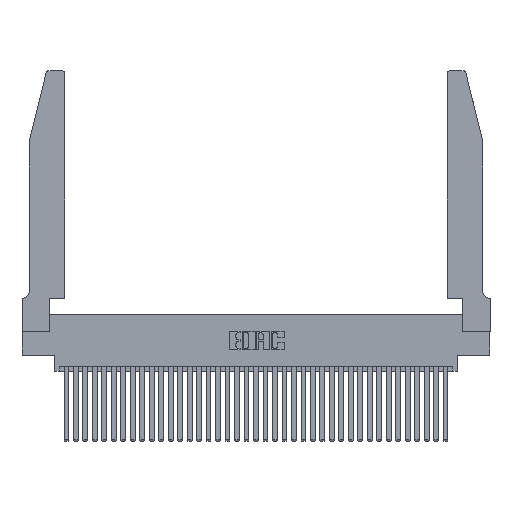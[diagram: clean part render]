
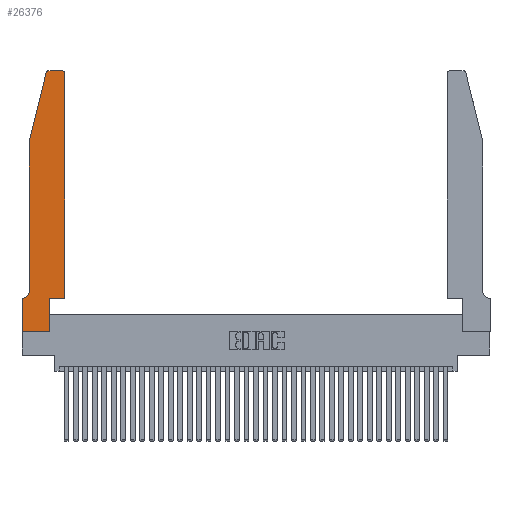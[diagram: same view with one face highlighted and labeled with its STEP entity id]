
A CAD part, top view. The second image highlights one B-rep face of the part: STEP entity #26376.
In plain terms, the highlighted planar face has unit normal (0, 0, 1).
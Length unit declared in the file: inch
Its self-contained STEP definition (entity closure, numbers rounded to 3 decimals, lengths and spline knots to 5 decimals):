
#1013 = VERTEX_POINT ( 'NONE', #22305 ) ;
#1268 = ORIENTED_EDGE ( 'NONE', *, *, #36997, .T. ) ;
#1729 = VERTEX_POINT ( 'NONE', #36439 ) ;
#1864 = DIRECTION ( 'NONE',  ( 0., 0., 1. ) ) ;
#2019 = EDGE_CURVE ( 'NONE', #1013, #4661, #13661, .T. ) ;
#2986 = VERTEX_POINT ( 'NONE', #23632 ) ;
#3375 = VERTEX_POINT ( 'NONE', #32459 ) ;
#4185 = VERTEX_POINT ( 'NONE', #5945 ) ;
#4413 = CARTESIAN_POINT ( 'NONE',  ( 0.0755, 0.42, 0.37 ) ) ;
#4527 = VECTOR ( 'NONE', #27788, 39.37008 ) ;
#4661 = VERTEX_POINT ( 'NONE', #18402 ) ;
#5236 = AXIS2_PLACEMENT_3D ( 'NONE', #10048, #24263, #25766 ) ;
#5722 = DIRECTION ( 'NONE',  ( 0., 1., 0. ) ) ;
#5833 = EDGE_CURVE ( 'NONE', #34220, #34343, #16683, .T. ) ;
#5945 = CARTESIAN_POINT ( 'NONE',  ( 0.4205, 2.75, 0.37 ) ) ;
#6060 = ORIENTED_EDGE ( 'NONE', *, *, #17076, .T. ) ;
#6767 = EDGE_CURVE ( 'NONE', #4185, #9011, #18855, .T. ) ;
#6875 = EDGE_CURVE ( 'NONE', #2986, #26471, #8984, .T. ) ;
#7191 = CARTESIAN_POINT ( 'NONE',  ( 0.4505, 2.72, 0.37 ) ) ;
#7419 = VECTOR ( 'NONE', #5722, 39.37008 ) ;
#8984 = LINE ( 'NONE', #25516, #24619 ) ;
#9011 = VERTEX_POINT ( 'NONE', #24114 ) ;
#9101 = EDGE_CURVE ( 'NONE', #26471, #4185, #30665, .T. ) ;
#9399 = EDGE_CURVE ( 'NONE', #3375, #12398, #28418, .T. ) ;
#9573 = DIRECTION ( 'NONE',  ( 1., 0., 0. ) ) ;
#9717 = CARTESIAN_POINT ( 'NONE',  ( 0.0055, 0.35, 0.37 ) ) ;
#10048 = CARTESIAN_POINT ( 'NONE',  ( 0.0055, 0.42, 0.37 ) ) ;
#10257 = CARTESIAN_POINT ( 'NONE',  ( 0., 0.35, 0.37 ) ) ;
#10322 = ORIENTED_EDGE ( 'NONE', *, *, #9101, .T. ) ;
#10904 = DIRECTION ( 'NONE',  ( 0., -1., 0. ) ) ;
#11221 = DIRECTION ( 'NONE',  ( 0., -1., 0. ) ) ;
#11680 = VECTOR ( 'NONE', #27856, 39.37008 ) ;
#12184 = FACE_OUTER_BOUND ( 'NONE', #31581, .T. ) ;
#12398 = VERTEX_POINT ( 'NONE', #4413 ) ;
#12645 = DIRECTION ( 'NONE',  ( 1., 0., 0. ) ) ;
#13221 = VECTOR ( 'NONE', #12645, 39.37008 ) ;
#13618 = ORIENTED_EDGE ( 'NONE', *, *, #2019, .T. ) ;
#13643 = CARTESIAN_POINT ( 'NONE',  ( 0.0755, 2., 0.37 ) ) ;
#13661 = LINE ( 'NONE', #36931, #7419 ) ;
#13960 = AXIS2_PLACEMENT_3D ( 'NONE', #15125, #35069, #20920 ) ;
#13975 = CARTESIAN_POINT ( 'NONE',  ( 0.0755, 2., 0.37 ) ) ;
#15125 = CARTESIAN_POINT ( 'NONE',  ( 0.4205, 2.72, 0.37 ) ) ;
#16138 = EDGE_CURVE ( 'NONE', #1729, #3375, #25161, .T. ) ;
#16359 = ORIENTED_EDGE ( 'NONE', *, *, #32297, .T. ) ;
#16491 = CARTESIAN_POINT ( 'NONE',  ( 0., 0., 0.37 ) ) ;
#16683 = LINE ( 'NONE', #28281, #29590 ) ;
#16897 = ORIENTED_EDGE ( 'NONE', *, *, #5833, .T. ) ;
#17048 = ORIENTED_EDGE ( 'NONE', *, *, #20225, .T. ) ;
#17060 = ORIENTED_EDGE ( 'NONE', *, *, #33007, .T. ) ;
#17076 = EDGE_CURVE ( 'NONE', #12398, #32740, #30425, .T. ) ;
#17325 = ORIENTED_EDGE ( 'NONE', *, *, #9399, .T. ) ;
#18003 = PLANE ( 'NONE',  #36859 ) ;
#18330 = CARTESIAN_POINT ( 'NONE',  ( 0.4505, 0.35, 0.37 ) ) ;
#18402 = CARTESIAN_POINT ( 'NONE',  ( 0.2865, 0.35, 0.37 ) ) ;
#18855 = LINE ( 'NONE', #27982, #11680 ) ;
#19780 = LINE ( 'NONE', #16491, #4527 ) ;
#19934 = DIRECTION ( 'NONE',  ( 0., 1., 0. ) ) ;
#20225 = EDGE_CURVE ( 'NONE', #32740, #34220, #25562, .T. ) ;
#20920 = DIRECTION ( 'NONE',  ( 1., 0., 0. ) ) ;
#21389 = CARTESIAN_POINT ( 'NONE',  ( 0.0755, 0.35, 0.37 ) ) ;
#21783 = CARTESIAN_POINT ( 'NONE',  ( 0.284, 2.72, 0.37 ) ) ;
#21964 = ORIENTED_EDGE ( 'NONE', *, *, #6875, .T. ) ;
#22305 = CARTESIAN_POINT ( 'NONE',  ( 0.2865, 0., 0.37 ) ) ;
#22685 = AXIS2_PLACEMENT_3D ( 'NONE', #21783, #1864, #33427 ) ;
#22883 = VECTOR ( 'NONE', #24108, 39.37008 ) ;
#23632 = CARTESIAN_POINT ( 'NONE',  ( 0.4505, 0.35, 0.37 ) ) ;
#24108 = DIRECTION ( 'NONE',  ( -1., 0., 0. ) ) ;
#24114 = CARTESIAN_POINT ( 'NONE',  ( 0.284, 2.75, 0.37 ) ) ;
#24263 = DIRECTION ( 'NONE',  ( 0., 0., -1. ) ) ;
#24619 = VECTOR ( 'NONE', #19934, 39.37008 ) ;
#25161 = LINE ( 'NONE', #13975, #34023 ) ;
#25516 = CARTESIAN_POINT ( 'NONE',  ( 0.4505, 0.35, 0.37 ) ) ;
#25562 = LINE ( 'NONE', #21389, #22883 ) ;
#25766 = DIRECTION ( 'NONE',  ( -1., 0., 0. ) ) ;
#26376 = ADVANCED_FACE ( 'NONE', ( #12184 ), #18003, .T. ) ;
#26471 = VERTEX_POINT ( 'NONE', #7191 ) ;
#27380 = CIRCLE ( 'NONE', #22685, 0.03 ) ;
#27534 = VECTOR ( 'NONE', #10904, 39.37008 ) ;
#27788 = DIRECTION ( 'NONE',  ( 1., 0., 0. ) ) ;
#27856 = DIRECTION ( 'NONE',  ( -1., 0., 0. ) ) ;
#27982 = CARTESIAN_POINT ( 'NONE',  ( 0.2605, 2.75, 0.37 ) ) ;
#28069 = ORIENTED_EDGE ( 'NONE', *, *, #16138, .T. ) ;
#28281 = CARTESIAN_POINT ( 'NONE',  ( 0., 0., 0.37 ) ) ;
#28311 = CARTESIAN_POINT ( 'NONE',  ( 0., 0., 0.37 ) ) ;
#28381 = LINE ( 'NONE', #18330, #13221 ) ;
#28418 = LINE ( 'NONE', #13643, #27534 ) ;
#29590 = VECTOR ( 'NONE', #11221, 39.37008 ) ;
#30425 = CIRCLE ( 'NONE', #5236, 0.07 ) ;
#30608 = ORIENTED_EDGE ( 'NONE', *, *, #6767, .T. ) ;
#30665 = CIRCLE ( 'NONE', #13960, 0.03 ) ;
#31581 = EDGE_LOOP ( 'NONE', ( #30608, #16359, #28069, #17325, #6060, #17048, #16897, #17060, #13618, #1268, #21964, #10322 ) ) ;
#32297 = EDGE_CURVE ( 'NONE', #9011, #1729, #27380, .T. ) ;
#32377 = CARTESIAN_POINT ( 'NONE',  ( 0., 0.35, 0.37 ) ) ;
#32459 = CARTESIAN_POINT ( 'NONE',  ( 0.0755, 2., 0.37 ) ) ;
#32740 = VERTEX_POINT ( 'NONE', #9717 ) ;
#33007 = EDGE_CURVE ( 'NONE', #34343, #1013, #19780, .T. ) ;
#33427 = DIRECTION ( 'NONE',  ( 1., 0., 0. ) ) ;
#34023 = VECTOR ( 'NONE', #34660, 39.37008 ) ;
#34220 = VERTEX_POINT ( 'NONE', #10257 ) ;
#34343 = VERTEX_POINT ( 'NONE', #28311 ) ;
#34660 = DIRECTION ( 'NONE',  ( -0.239, -0.971, 0. ) ) ;
#35069 = DIRECTION ( 'NONE',  ( 0., 0., 1. ) ) ;
#35394 = DIRECTION ( 'NONE',  ( 0., 0., 1. ) ) ;
#36439 = CARTESIAN_POINT ( 'NONE',  ( 0.25487, 2.72718, 0.37 ) ) ;
#36859 = AXIS2_PLACEMENT_3D ( 'NONE', #32377, #35394, #9573 ) ;
#36931 = CARTESIAN_POINT ( 'NONE',  ( 0.2865, 0.35, 0.37 ) ) ;
#36997 = EDGE_CURVE ( 'NONE', #4661, #2986, #28381, .T. ) ;
